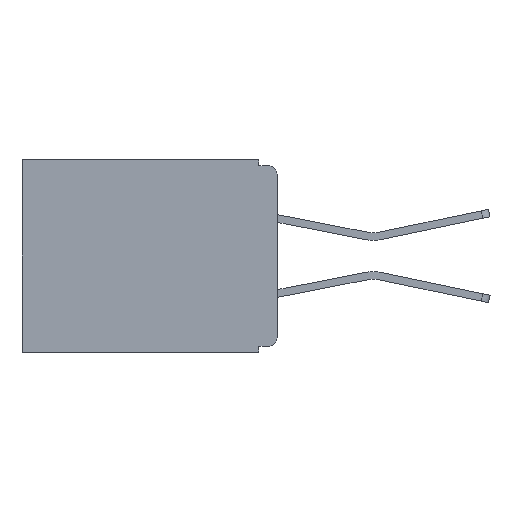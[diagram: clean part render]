
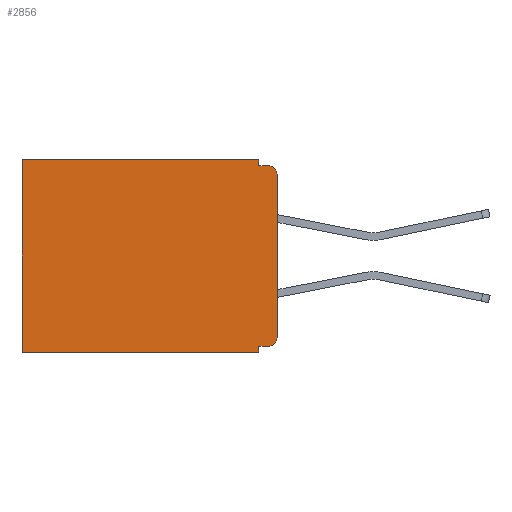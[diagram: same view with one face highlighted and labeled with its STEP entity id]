
A CAD part, left-side view. The second image highlights one B-rep face of the part: STEP entity #2856.
In plain terms, the highlighted planar face has unit normal (-1, 0, 0).
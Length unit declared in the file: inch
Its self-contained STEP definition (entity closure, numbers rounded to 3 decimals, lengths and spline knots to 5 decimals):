
#25 = DIRECTION ( 'NONE',  ( 0., 1., 0. ) ) ;
#43 = CARTESIAN_POINT ( 'NONE',  ( 0.3, 0.015, -0.01 ) ) ;
#514 = CARTESIAN_POINT ( 'NONE',  ( 0.3, 0., -0.01 ) ) ;
#531 = LINE ( 'NONE', #10883, #13169 ) ;
#600 = DIRECTION ( 'NONE',  ( 0., 0., -1. ) ) ;
#933 = VECTOR ( 'NONE', #25, 39.37008 ) ;
#1059 = DIRECTION ( 'NONE',  ( 0., 0., -1. ) ) ;
#1087 = VERTEX_POINT ( 'NONE', #5595 ) ;
#1108 = VERTEX_POINT ( 'NONE', #5951 ) ;
#1165 = VECTOR ( 'NONE', #4822, 39.37008 ) ;
#1299 = VECTOR ( 'NONE', #12310, 39.37008 ) ;
#1398 = CIRCLE ( 'NONE', #2237, 0.015 ) ;
#1578 = LINE ( 'NONE', #8623, #1165 ) ;
#1984 = DIRECTION ( 'NONE',  ( 0., 0., -1. ) ) ;
#1994 = CARTESIAN_POINT ( 'NONE',  ( 0.3, 0., -0.305 ) ) ;
#2237 = AXIS2_PLACEMENT_3D ( 'NONE', #9296, #3516, #1984 ) ;
#2255 = EDGE_CURVE ( 'NONE', #12380, #7812, #1398, .T. ) ;
#2281 = EDGE_CURVE ( 'NONE', #15080, #15888, #531, .T. ) ;
#2542 = LINE ( 'NONE', #514, #8960 ) ;
#2856 = ADVANCED_FACE ( 'NONE', ( #4689 ), #10099, .F. ) ;
#3174 = DIRECTION ( 'NONE',  ( 0., -1., 0. ) ) ;
#3282 = ORIENTED_EDGE ( 'NONE', *, *, #9048, .T. ) ;
#3317 = DIRECTION ( 'NONE',  ( -1., 0., 0. ) ) ;
#3516 = DIRECTION ( 'NONE',  ( -1., 0., 0. ) ) ;
#4115 = VERTEX_POINT ( 'NONE', #4740 ) ;
#4217 = VERTEX_POINT ( 'NONE', #10688 ) ;
#4689 = FACE_OUTER_BOUND ( 'NONE', #14470, .T. ) ;
#4740 = CARTESIAN_POINT ( 'NONE',  ( 0.3, 0.015, -0.32 ) ) ;
#4822 = DIRECTION ( 'NONE',  ( 0., 0., -1. ) ) ;
#5175 = ORIENTED_EDGE ( 'NONE', *, *, #14540, .T. ) ;
#5587 = DIRECTION ( 'NONE',  ( 0., 1., 0. ) ) ;
#5595 = CARTESIAN_POINT ( 'NONE',  ( 0.3, 0.437, -0.33 ) ) ;
#5650 = ORIENTED_EDGE ( 'NONE', *, *, #15974, .F. ) ;
#5951 = CARTESIAN_POINT ( 'NONE',  ( 0.3, 0.031, -0.33 ) ) ;
#5983 = ORIENTED_EDGE ( 'NONE', *, *, #2281, .F. ) ;
#5994 = AXIS2_PLACEMENT_3D ( 'NONE', #9120, #15585, #1059 ) ;
#6083 = CARTESIAN_POINT ( 'NONE',  ( 0.3, 0., -0.33 ) ) ;
#6395 = CIRCLE ( 'NONE', #12432, 0.015 ) ;
#6966 = VECTOR ( 'NONE', #600, 39.37008 ) ;
#7237 = CARTESIAN_POINT ( 'NONE',  ( 0.3, 0.437, 0. ) ) ;
#7642 = CARTESIAN_POINT ( 'NONE',  ( 0.3, 0.031, 0. ) ) ;
#7812 = VERTEX_POINT ( 'NONE', #43 ) ;
#7968 = ORIENTED_EDGE ( 'NONE', *, *, #8921, .T. ) ;
#8171 = LINE ( 'NONE', #11112, #1299 ) ;
#8623 = CARTESIAN_POINT ( 'NONE',  ( 0.3, 0.031, -0.33 ) ) ;
#8921 = EDGE_CURVE ( 'NONE', #4115, #14195, #6395, .T. ) ;
#8960 = VECTOR ( 'NONE', #3174, 39.37008 ) ;
#8992 = LINE ( 'NONE', #13829, #933 ) ;
#9048 = EDGE_CURVE ( 'NONE', #10082, #1087, #8171, .T. ) ;
#9105 = LINE ( 'NONE', #6083, #10643 ) ;
#9120 = CARTESIAN_POINT ( 'NONE',  ( 0.3, 0., -0.33 ) ) ;
#9296 = CARTESIAN_POINT ( 'NONE',  ( 0.3, 0.015, -0.025 ) ) ;
#9377 = CARTESIAN_POINT ( 'NONE',  ( 0.3, 0.031, -0.01 ) ) ;
#9499 = EDGE_CURVE ( 'NONE', #12380, #14195, #10236, .T. ) ;
#9590 = EDGE_CURVE ( 'NONE', #1108, #1087, #9105, .T. ) ;
#9600 = LINE ( 'NONE', #15326, #12424 ) ;
#9847 = ORIENTED_EDGE ( 'NONE', *, *, #9499, .F. ) ;
#10035 = ORIENTED_EDGE ( 'NONE', *, *, #13790, .F. ) ;
#10082 = VERTEX_POINT ( 'NONE', #7237 ) ;
#10099 = PLANE ( 'NONE',  #5994 ) ;
#10236 = LINE ( 'NONE', #11990, #6966 ) ;
#10382 = DIRECTION ( 'NONE',  ( 0., 0., -1. ) ) ;
#10643 = VECTOR ( 'NONE', #14593, 39.37008 ) ;
#10688 = CARTESIAN_POINT ( 'NONE',  ( 0.3, 0.031, -0.32 ) ) ;
#10850 = ORIENTED_EDGE ( 'NONE', *, *, #14300, .F. ) ;
#10883 = CARTESIAN_POINT ( 'NONE',  ( 0.3, 0.031, 0. ) ) ;
#10915 = CARTESIAN_POINT ( 'NONE',  ( 0.3, 0.015, -0.305 ) ) ;
#11112 = CARTESIAN_POINT ( 'NONE',  ( 0.3, 0.437, -0.33 ) ) ;
#11990 = CARTESIAN_POINT ( 'NONE',  ( 0.3, 0., -0.33 ) ) ;
#12112 = DIRECTION ( 'NONE',  ( 0., 0., -1. ) ) ;
#12310 = DIRECTION ( 'NONE',  ( 0., 0., -1. ) ) ;
#12380 = VERTEX_POINT ( 'NONE', #15003 ) ;
#12424 = VECTOR ( 'NONE', #5587, 39.37008 ) ;
#12432 = AXIS2_PLACEMENT_3D ( 'NONE', #10915, #3317, #12112 ) ;
#13169 = VECTOR ( 'NONE', #10382, 39.37008 ) ;
#13790 = EDGE_CURVE ( 'NONE', #4115, #4217, #9600, .T. ) ;
#13829 = CARTESIAN_POINT ( 'NONE',  ( 0.3, 0., 0. ) ) ;
#14195 = VERTEX_POINT ( 'NONE', #1994 ) ;
#14300 = EDGE_CURVE ( 'NONE', #4217, #1108, #1578, .T. ) ;
#14470 = EDGE_LOOP ( 'NONE', ( #9847, #14561, #5650, #5983, #5175, #3282, #15678, #10850, #10035, #7968 ) ) ;
#14540 = EDGE_CURVE ( 'NONE', #15080, #10082, #8992, .T. ) ;
#14561 = ORIENTED_EDGE ( 'NONE', *, *, #2255, .T. ) ;
#14593 = DIRECTION ( 'NONE',  ( 0., 1., 0. ) ) ;
#15003 = CARTESIAN_POINT ( 'NONE',  ( 0.3, 0., -0.025 ) ) ;
#15080 = VERTEX_POINT ( 'NONE', #7642 ) ;
#15326 = CARTESIAN_POINT ( 'NONE',  ( 0.3, 0., -0.32 ) ) ;
#15585 = DIRECTION ( 'NONE',  ( 1., 0., 0. ) ) ;
#15678 = ORIENTED_EDGE ( 'NONE', *, *, #9590, .F. ) ;
#15888 = VERTEX_POINT ( 'NONE', #9377 ) ;
#15974 = EDGE_CURVE ( 'NONE', #15888, #7812, #2542, .T. ) ;
